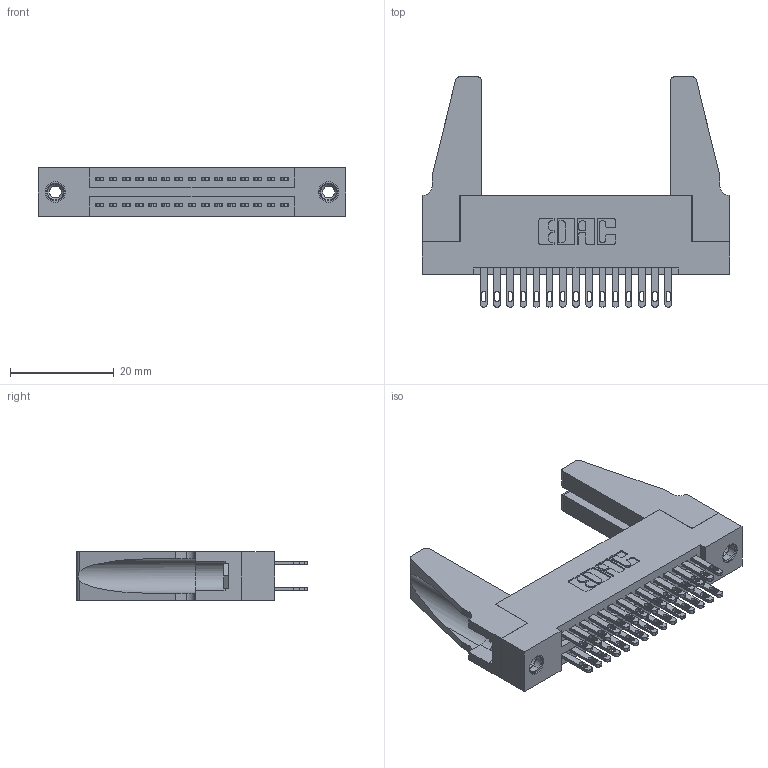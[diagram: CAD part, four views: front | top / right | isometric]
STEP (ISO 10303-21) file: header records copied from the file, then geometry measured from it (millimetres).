
FILE_DESCRIPTION (( 'STEP AP203' ), '1' );
FILE_NAME ('345-030-500-288.STEP', '2019-10-28T01:03:29', ( '' ), ( '' ), 'SwSTEP 2.0', 'SolidWorks 2016', '' );
FILE_SCHEMA (( 'CONFIG_CONTROL_DESIGN' ));
Length unit declared in the file: inch
Products named in the file (5): 345-030-500-288; 345-250-001_345-250-001-102; 345-292-001_345-293-100; 345 Part_Flush Mounting Lugs - 0.156 Dia-TH; 345-220-078_345-220-088
Assembly tree (35 placements, depth 2):
  345-030-500-288
    345 Part_Flush Mounting Lugs - 0.156 Dia-TH
    345-292-001_345-293-100  x30
    345-250-001_345-250-001-102  x2
    345-220-078_345-220-088  x2
Bounding box: 59.33 x 44.37 x 9.4 mm (x, y, z)
Volume: 8857.3 mm3; surface area: 11190.1 mm2
Topology: 35 solids, 35 shells, 1630 faces, 4885 edges, 3246 vertices
Faces by surface type: plane 962, cylinder 652, cone 12, torus 4
Entity records: 17482 total; most frequent: CARTESIAN_POINT 2950, ORIENTED_EDGE 2844, DIRECTION 2642, EDGE_CURVE 1422, LINE 1184, VECTOR 1184, VERTEX_POINT 942, AXIS2_PLACEMENT_3D 729
